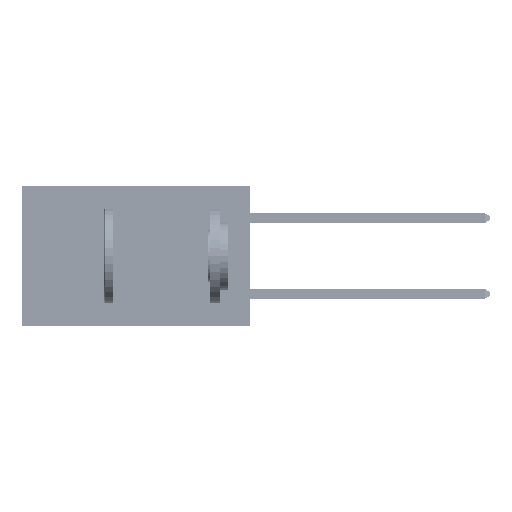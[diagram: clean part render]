
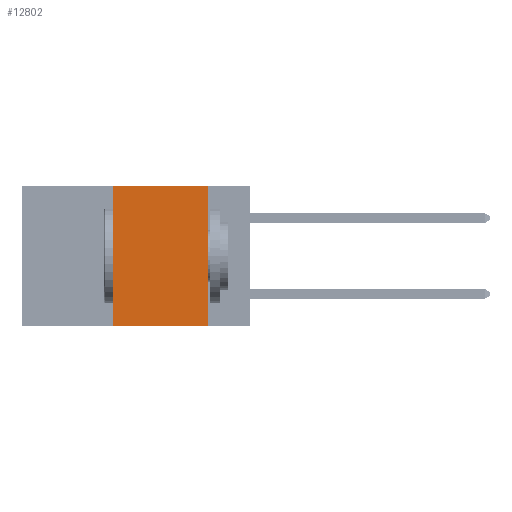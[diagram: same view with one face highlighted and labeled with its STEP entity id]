
A CAD part, left-side view. The second image highlights one B-rep face of the part: STEP entity #12802.
In plain terms, the highlighted planar face has unit normal (-1, 0, 0).
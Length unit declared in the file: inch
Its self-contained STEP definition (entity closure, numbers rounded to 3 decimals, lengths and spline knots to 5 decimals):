
#1139 = EDGE_CURVE ( 'NONE', #35380, #7330, #3507, .T. ) ;
#2488 = CARTESIAN_POINT ( 'NONE',  ( 0., 0.6, 0. ) ) ;
#2771 = ORIENTED_EDGE ( 'NONE', *, *, #5160, .F. ) ;
#2789 = EDGE_LOOP ( 'NONE', ( #2771, #10915, #35176, #49442 ) ) ;
#2815 = CARTESIAN_POINT ( 'NONE',  ( 0., 0.11, 0. ) ) ;
#3507 = LINE ( 'NONE', #10425, #21792 ) ;
#5160 = EDGE_CURVE ( 'NONE', #42405, #7330, #5757, .T. ) ;
#5757 = LINE ( 'NONE', #2815, #26442 ) ;
#5963 = FACE_OUTER_BOUND ( 'NONE', #2789, .T. ) ;
#6430 = DIRECTION ( 'NONE',  ( 0., 0., -1. ) ) ;
#7330 = VERTEX_POINT ( 'NONE', #25561 ) ;
#8105 = EDGE_CURVE ( 'NONE', #35380, #28818, #45930, .T. ) ;
#9900 = VECTOR ( 'NONE', #49502, 39.37008 ) ;
#10425 = CARTESIAN_POINT ( 'NONE',  ( 0., 0.6, -0.37 ) ) ;
#10476 = EDGE_CURVE ( 'NONE', #28818, #42405, #40763, .T. ) ;
#10915 = ORIENTED_EDGE ( 'NONE', *, *, #10476, .F. ) ;
#12802 = ADVANCED_FACE ( 'NONE', ( #5963 ), #37324, .F. ) ;
#16026 = CARTESIAN_POINT ( 'NONE',  ( 0., 0.36, 0. ) ) ;
#16088 = CARTESIAN_POINT ( 'NONE',  ( 0., 0.11, 0. ) ) ;
#18226 = DIRECTION ( 'NONE',  ( 0., -1., 0. ) ) ;
#18812 = CARTESIAN_POINT ( 'NONE',  ( 0., 0.6, 0. ) ) ;
#21792 = VECTOR ( 'NONE', #18226, 39.37008 ) ;
#22109 = CARTESIAN_POINT ( 'NONE',  ( 0., 0.36, 0. ) ) ;
#25561 = CARTESIAN_POINT ( 'NONE',  ( 0., 0.11, -0.37 ) ) ;
#25990 = DIRECTION ( 'NONE',  ( 0., 0., 1. ) ) ;
#26144 = DIRECTION ( 'NONE',  ( 0., 0., -1. ) ) ;
#26442 = VECTOR ( 'NONE', #26144, 39.37008 ) ;
#28818 = VERTEX_POINT ( 'NONE', #16026 ) ;
#29720 = DIRECTION ( 'NONE',  ( 1., 0., 0. ) ) ;
#33441 = AXIS2_PLACEMENT_3D ( 'NONE', #2488, #29720, #6430 ) ;
#35176 = ORIENTED_EDGE ( 'NONE', *, *, #8105, .F. ) ;
#35380 = VERTEX_POINT ( 'NONE', #42220 ) ;
#35803 = VECTOR ( 'NONE', #25990, 39.37008 ) ;
#37324 = PLANE ( 'NONE',  #33441 ) ;
#40763 = LINE ( 'NONE', #18812, #9900 ) ;
#42220 = CARTESIAN_POINT ( 'NONE',  ( 0., 0.36, -0.37 ) ) ;
#42405 = VERTEX_POINT ( 'NONE', #16088 ) ;
#45930 = LINE ( 'NONE', #22109, #35803 ) ;
#49442 = ORIENTED_EDGE ( 'NONE', *, *, #1139, .T. ) ;
#49502 = DIRECTION ( 'NONE',  ( 0., -1., 0. ) ) ;
